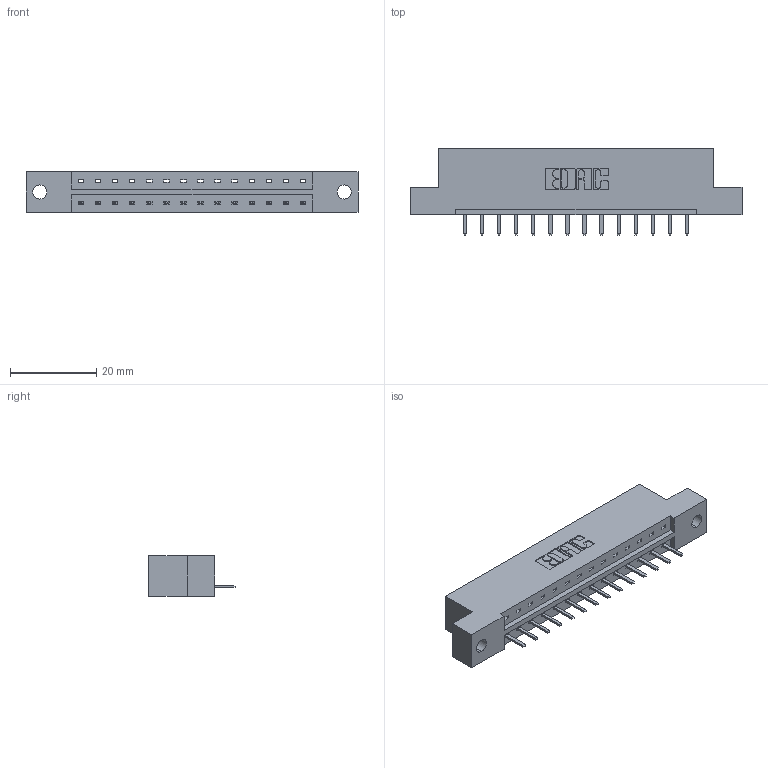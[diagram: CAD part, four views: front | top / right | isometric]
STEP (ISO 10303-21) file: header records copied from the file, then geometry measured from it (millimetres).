
FILE_DESCRIPTION (( 'STEP AP203' ), '1' );
FILE_NAME ('333-014-520-102.STEP', '2018-08-01T01:52:49', ( '' ), ( '' ), 'SwSTEP 2.0', 'SolidWorks 2016', '' );
FILE_SCHEMA (( 'CONFIG_CONTROL_DESIGN' ));
Length unit declared in the file: inch
Products named in the file (3): 333 Part_Flush - .128 Dia; 345-292-001_345-293-120; 333-014-520-102
Assembly tree (15 placements, depth 2):
  333-014-520-102
    333 Part_Flush - .128 Dia
    345-292-001_345-293-120  x14
Bounding box: 77.01 x 20.02 x 9.4 mm (x, y, z)
Volume: 7431.9 mm3; surface area: 7444.4 mm2
Topology: 15 solids, 15 shells, 982 faces, 2887 edges, 1886 vertices
Faces by surface type: plane 686, cylinder 296
Entity records: 12297 total; most frequent: CARTESIAN_POINT 2144, ORIENTED_EDGE 2082, DIRECTION 1853, EDGE_CURVE 1041, LINE 909, VECTOR 909, VERTEX_POINT 690, AXIS2_PLACEMENT_3D 472
